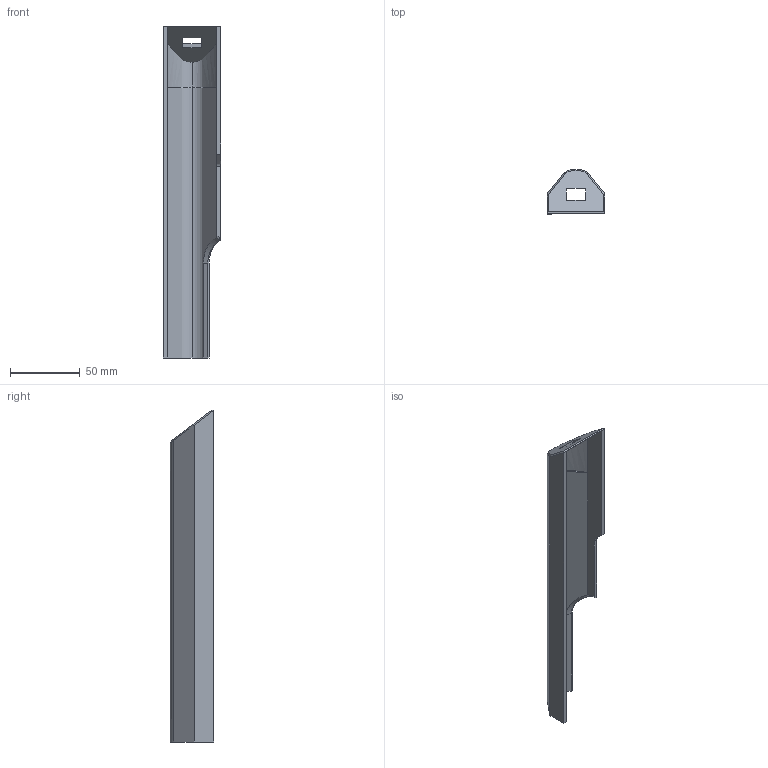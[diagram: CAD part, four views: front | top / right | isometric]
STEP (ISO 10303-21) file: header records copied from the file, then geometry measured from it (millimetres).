
FILE_DESCRIPTION(/* description */ (''),/* implementation_level */ '2;1');
FILE_NAME(/* name */ 'Printed Dust Cover - Plain.stp',/* time_stamp */ '2020-09-06T11:46:27-05:00',/* author */ ('johne'),/* organization */ (''),/* preprocessor_version */ 'ST-DEVELOPER v18',/* originating_system */ 'Autodesk Inventor 2020',/* authorisation */ '');
FILE_SCHEMA (('AUTOMOTIVE_DESIGN { 1 0 10303 214 3 1 1 }'));
Length unit declared in the file: millimetre
Products named in the file (1): Upper Receiver Cover
Bounding box: 41.43 x 31.35 x 237.3 mm (x, y, z)
Volume: 38500.5 mm3; surface area: 34632.7 mm2
Topology: 1 solids, 1 shells, 52 faces, 144 edges, 94 vertices
Faces by surface type: plane 32, cylinder 14, cone 3, bspline 3
Entity records: 1854 total; most frequent: CARTESIAN_POINT 486, ORIENTED_EDGE 288, DIRECTION 259, EDGE_CURVE 144, VERTEX_POINT 94, LINE 89, VECTOR 89, AXIS2_PLACEMENT_3D 85
